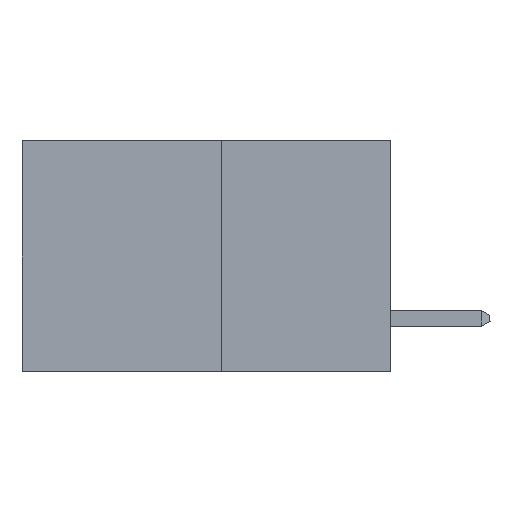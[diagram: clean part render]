
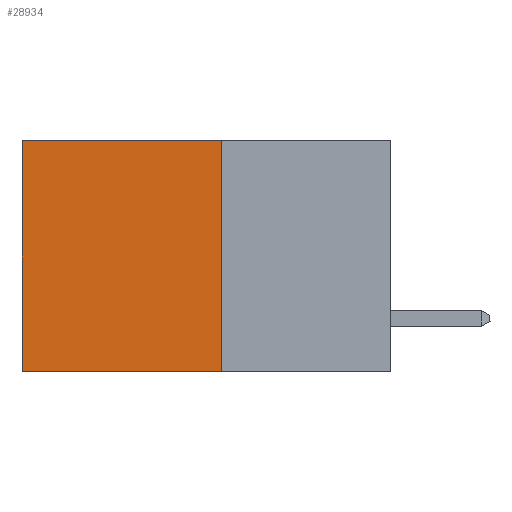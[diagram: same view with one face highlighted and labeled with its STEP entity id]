
A CAD part, left-side view. The second image highlights one B-rep face of the part: STEP entity #28934.
In plain terms, the highlighted planar face has unit normal (-1, 0, 0).
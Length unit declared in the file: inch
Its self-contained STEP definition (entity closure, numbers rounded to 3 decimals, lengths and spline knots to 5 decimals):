
#598 = VERTEX_POINT ( 'NONE', #29445 ) ;
#650 = VERTEX_POINT ( 'NONE', #26415 ) ;
#1569 = EDGE_CURVE ( 'NONE', #650, #598, #18633, .T. ) ;
#2264 = EDGE_LOOP ( 'NONE', ( #10809, #5106, #15808, #10701 ) ) ;
#4171 = LINE ( 'NONE', #17285, #16699 ) ;
#5106 = ORIENTED_EDGE ( 'NONE', *, *, #20452, .F. ) ;
#8000 = CARTESIAN_POINT ( 'NONE',  ( 0.277, 0.27, -0.37 ) ) ;
#9329 = VERTEX_POINT ( 'NONE', #21169 ) ;
#9536 = VECTOR ( 'NONE', #30050, 39.37008 ) ;
#10523 = DIRECTION ( 'NONE',  ( 0., 0., -1. ) ) ;
#10701 = ORIENTED_EDGE ( 'NONE', *, *, #17769, .T. ) ;
#10809 = ORIENTED_EDGE ( 'NONE', *, *, #1569, .T. ) ;
#14463 = EDGE_CURVE ( 'NONE', #23679, #9329, #29209, .T. ) ;
#15808 = ORIENTED_EDGE ( 'NONE', *, *, #14463, .F. ) ;
#16306 = FACE_OUTER_BOUND ( 'NONE', #2264, .T. ) ;
#16699 = VECTOR ( 'NONE', #19748, 39.37008 ) ;
#17285 = CARTESIAN_POINT ( 'NONE',  ( 0.277, 0.27, -0.37 ) ) ;
#17769 = EDGE_CURVE ( 'NONE', #23679, #650, #26824, .T. ) ;
#17873 = DIRECTION ( 'NONE',  ( 0., 0., -1. ) ) ;
#18079 = CARTESIAN_POINT ( 'NONE',  ( 0.277, 0.59, -0.37 ) ) ;
#18633 = LINE ( 'NONE', #18079, #30883 ) ;
#19748 = DIRECTION ( 'NONE',  ( 0., 1., 0. ) ) ;
#20312 = VECTOR ( 'NONE', #24020, 39.37008 ) ;
#20452 = EDGE_CURVE ( 'NONE', #9329, #598, #4171, .T. ) ;
#21169 = CARTESIAN_POINT ( 'NONE',  ( 0.277, 0.27, -0.37 ) ) ;
#21602 = CARTESIAN_POINT ( 'NONE',  ( 0.277, 0.27, 0. ) ) ;
#22899 = PLANE ( 'NONE',  #23382 ) ;
#23382 = AXIS2_PLACEMENT_3D ( 'NONE', #8000, #25298, #10523 ) ;
#23679 = VERTEX_POINT ( 'NONE', #28482 ) ;
#24020 = DIRECTION ( 'NONE',  ( 0., 1., 0. ) ) ;
#25298 = DIRECTION ( 'NONE',  ( 1., 0., 0. ) ) ;
#26415 = CARTESIAN_POINT ( 'NONE',  ( 0.277, 0.59, 0. ) ) ;
#26824 = LINE ( 'NONE', #21602, #20312 ) ;
#27591 = CARTESIAN_POINT ( 'NONE',  ( 0.277, 0.27, -0.37 ) ) ;
#28482 = CARTESIAN_POINT ( 'NONE',  ( 0.277, 0.27, 0. ) ) ;
#28934 = ADVANCED_FACE ( 'NONE', ( #16306 ), #22899, .F. ) ;
#29209 = LINE ( 'NONE', #27591, #9536 ) ;
#29445 = CARTESIAN_POINT ( 'NONE',  ( 0.277, 0.59, -0.37 ) ) ;
#30050 = DIRECTION ( 'NONE',  ( 0., 0., -1. ) ) ;
#30883 = VECTOR ( 'NONE', #17873, 39.37008 ) ;
